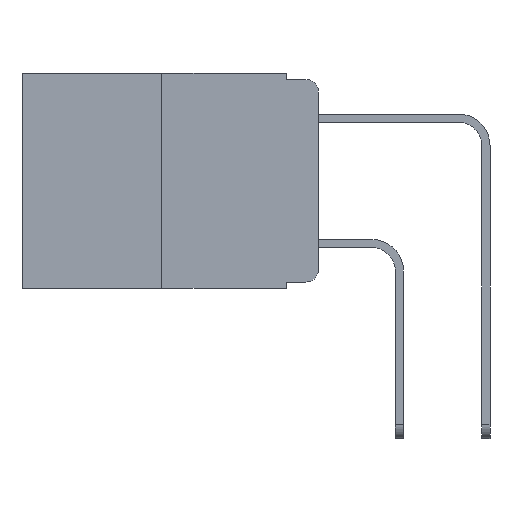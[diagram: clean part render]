
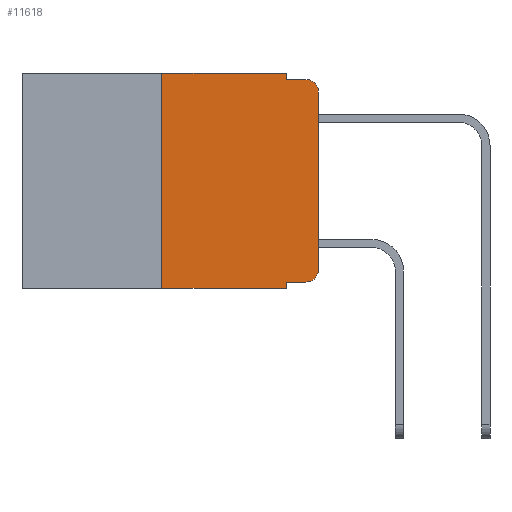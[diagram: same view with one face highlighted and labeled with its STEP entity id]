
A CAD part, left-side view. The second image highlights one B-rep face of the part: STEP entity #11618.
In plain terms, the highlighted planar face has unit normal (-1, 0, 0).
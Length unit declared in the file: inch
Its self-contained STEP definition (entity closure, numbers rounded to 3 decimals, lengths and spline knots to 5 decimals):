
#153 = ORIENTED_EDGE ( 'NONE', *, *, #5348, .T. ) ;
#198 = LINE ( 'NONE', #15571, #12559 ) ;
#219 = DIRECTION ( 'NONE',  ( -1., 0., 0. ) ) ;
#257 = VERTEX_POINT ( 'NONE', #8439 ) ;
#318 = VECTOR ( 'NONE', #11816, 39.37008 ) ;
#355 = DIRECTION ( 'NONE',  ( 0., 0., -1. ) ) ;
#421 = CARTESIAN_POINT ( 'NONE',  ( 0., 0.051, -0.01 ) ) ;
#467 = EDGE_CURVE ( 'NONE', #1305, #14634, #198, .T. ) ;
#572 = ORIENTED_EDGE ( 'NONE', *, *, #12344, .F. ) ;
#992 = DIRECTION ( 'NONE',  ( 0., 0., 1. ) ) ;
#1305 = VERTEX_POINT ( 'NONE', #6108 ) ;
#1956 = CIRCLE ( 'NONE', #10327, 0.02 ) ;
#2284 = CARTESIAN_POINT ( 'NONE',  ( 0., 0.051, -0.343 ) ) ;
#2312 = ORIENTED_EDGE ( 'NONE', *, *, #13126, .F. ) ;
#2677 = FACE_OUTER_BOUND ( 'NONE', #8923, .T. ) ;
#2970 = CARTESIAN_POINT ( 'NONE',  ( 0., 0.473, 0. ) ) ;
#3062 = ORIENTED_EDGE ( 'NONE', *, *, #9602, .F. ) ;
#3219 = VECTOR ( 'NONE', #13721, 39.37008 ) ;
#3259 = VERTEX_POINT ( 'NONE', #4727 ) ;
#3291 = LINE ( 'NONE', #7677, #15582 ) ;
#3710 = VERTEX_POINT ( 'NONE', #9109 ) ;
#3883 = LINE ( 'NONE', #10652, #318 ) ;
#4254 = CARTESIAN_POINT ( 'NONE',  ( 0., 0.051, 0. ) ) ;
#4345 = ORIENTED_EDGE ( 'NONE', *, *, #7588, .T. ) ;
#4382 = DIRECTION ( 'NONE',  ( 0., -1., 0. ) ) ;
#4630 = VERTEX_POINT ( 'NONE', #9527 ) ;
#4727 = CARTESIAN_POINT ( 'NONE',  ( 0., 0.051, -0.333 ) ) ;
#5113 = VERTEX_POINT ( 'NONE', #11422 ) ;
#5211 = CARTESIAN_POINT ( 'NONE',  ( 0., 0.25, 0. ) ) ;
#5348 = EDGE_CURVE ( 'NONE', #4630, #8927, #3883, .T. ) ;
#6039 = DIRECTION ( 'NONE',  ( 0., -1., 0. ) ) ;
#6108 = CARTESIAN_POINT ( 'NONE',  ( 0., 0., -0.313 ) ) ;
#6310 = CIRCLE ( 'NONE', #14343, 0.02 ) ;
#6351 = LINE ( 'NONE', #12715, #15402 ) ;
#6465 = ORIENTED_EDGE ( 'NONE', *, *, #9183, .T. ) ;
#6516 = VECTOR ( 'NONE', #992, 39.37008 ) ;
#6653 = DIRECTION ( 'NONE',  ( 1., 0., 0. ) ) ;
#6814 = DIRECTION ( 'NONE',  ( 0., 0., -1. ) ) ;
#6914 = CARTESIAN_POINT ( 'NONE',  ( 0., 0., -0.03 ) ) ;
#6979 = ORIENTED_EDGE ( 'NONE', *, *, #10793, .F. ) ;
#7588 = EDGE_CURVE ( 'NONE', #13089, #1305, #6310, .T. ) ;
#7677 = CARTESIAN_POINT ( 'NONE',  ( 0., 0.051, -0.333 ) ) ;
#7817 = CARTESIAN_POINT ( 'NONE',  ( 0., 0.02, -0.03 ) ) ;
#7906 = DIRECTION ( 'NONE',  ( -1., 0., 0. ) ) ;
#8439 = CARTESIAN_POINT ( 'NONE',  ( 0., 0.02, -0.01 ) ) ;
#8479 = CARTESIAN_POINT ( 'NONE',  ( 0., 0.25, 0. ) ) ;
#8923 = EDGE_LOOP ( 'NONE', ( #12278, #11850, #2312, #572, #3062, #6979, #153, #10160, #6465, #4345 ) ) ;
#8927 = VERTEX_POINT ( 'NONE', #2284 ) ;
#9027 = DIRECTION ( 'NONE',  ( 0., 0., -1. ) ) ;
#9085 = VECTOR ( 'NONE', #4382, 39.37008 ) ;
#9109 = CARTESIAN_POINT ( 'NONE',  ( 0., 0.051, 0. ) ) ;
#9183 = EDGE_CURVE ( 'NONE', #3259, #13089, #3291, .T. ) ;
#9186 = LINE ( 'NONE', #9615, #11945 ) ;
#9490 = AXIS2_PLACEMENT_3D ( 'NONE', #2970, #6653, #14906 ) ;
#9527 = CARTESIAN_POINT ( 'NONE',  ( 0., 0.25, -0.343 ) ) ;
#9602 = EDGE_CURVE ( 'NONE', #10347, #3710, #9186, .T. ) ;
#9615 = CARTESIAN_POINT ( 'NONE',  ( 0., 0.473, 0. ) ) ;
#9683 = LINE ( 'NONE', #4254, #3219 ) ;
#10022 = EDGE_CURVE ( 'NONE', #3259, #8927, #6351, .T. ) ;
#10160 = ORIENTED_EDGE ( 'NONE', *, *, #10022, .F. ) ;
#10327 = AXIS2_PLACEMENT_3D ( 'NONE', #7817, #219, #9027 ) ;
#10347 = VERTEX_POINT ( 'NONE', #5211 ) ;
#10652 = CARTESIAN_POINT ( 'NONE',  ( 0., 0.473, -0.343 ) ) ;
#10793 = EDGE_CURVE ( 'NONE', #4630, #10347, #12451, .T. ) ;
#11422 = CARTESIAN_POINT ( 'NONE',  ( 0., 0.051, -0.01 ) ) ;
#11618 = ADVANCED_FACE ( 'NONE', ( #2677 ), #13734, .F. ) ;
#11816 = DIRECTION ( 'NONE',  ( 0., -1., 0. ) ) ;
#11850 = ORIENTED_EDGE ( 'NONE', *, *, #13894, .T. ) ;
#11945 = VECTOR ( 'NONE', #6039, 39.37008 ) ;
#12219 = LINE ( 'NONE', #421, #9085 ) ;
#12278 = ORIENTED_EDGE ( 'NONE', *, *, #467, .T. ) ;
#12344 = EDGE_CURVE ( 'NONE', #3710, #5113, #9683, .T. ) ;
#12451 = LINE ( 'NONE', #8479, #6516 ) ;
#12559 = VECTOR ( 'NONE', #13485, 39.37008 ) ;
#12631 = CARTESIAN_POINT ( 'NONE',  ( 0., 0.02, -0.333 ) ) ;
#12715 = CARTESIAN_POINT ( 'NONE',  ( 0., 0.051, 0. ) ) ;
#13089 = VERTEX_POINT ( 'NONE', #12631 ) ;
#13126 = EDGE_CURVE ( 'NONE', #5113, #257, #12219, .T. ) ;
#13485 = DIRECTION ( 'NONE',  ( 0., 0., 1. ) ) ;
#13721 = DIRECTION ( 'NONE',  ( 0., 0., -1. ) ) ;
#13734 = PLANE ( 'NONE',  #9490 ) ;
#13894 = EDGE_CURVE ( 'NONE', #14634, #257, #1956, .T. ) ;
#14343 = AXIS2_PLACEMENT_3D ( 'NONE', #14963, #7906, #355 ) ;
#14634 = VERTEX_POINT ( 'NONE', #6914 ) ;
#14730 = DIRECTION ( 'NONE',  ( 0., -1., 0. ) ) ;
#14906 = DIRECTION ( 'NONE',  ( 0., 0., -1. ) ) ;
#14963 = CARTESIAN_POINT ( 'NONE',  ( 0., 0.02, -0.313 ) ) ;
#15402 = VECTOR ( 'NONE', #6814, 39.37008 ) ;
#15571 = CARTESIAN_POINT ( 'NONE',  ( 0., 0., 0. ) ) ;
#15582 = VECTOR ( 'NONE', #14730, 39.37008 ) ;
